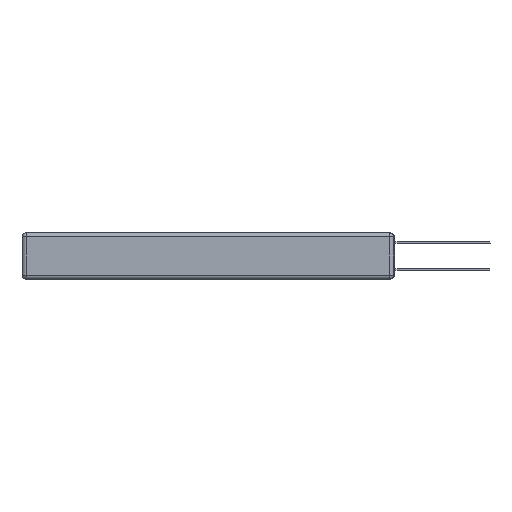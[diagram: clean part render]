
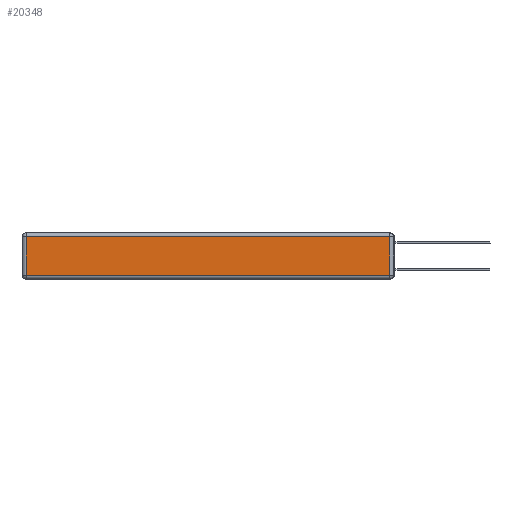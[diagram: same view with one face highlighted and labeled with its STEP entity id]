
A CAD part, left-side view. The second image highlights one B-rep face of the part: STEP entity #20348.
In plain terms, the highlighted planar face has unit normal (-1, 0, 0).
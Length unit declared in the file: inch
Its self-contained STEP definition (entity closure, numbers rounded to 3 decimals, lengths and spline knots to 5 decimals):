
#201 = VERTEX_POINT ( 'NONE', #10310 ) ;
#242 = VECTOR ( 'NONE', #2855, 39.37008 ) ;
#1112 = DIRECTION ( 'NONE',  ( 0., 0., -1. ) ) ;
#1991 = DIRECTION ( 'NONE',  ( 0., -1., 0. ) ) ;
#2254 = DIRECTION ( 'NONE',  ( 0., 0., 1. ) ) ;
#2322 = DIRECTION ( 'NONE',  ( -1., 0., 0. ) ) ;
#2855 = DIRECTION ( 'NONE',  ( 0., 0., 1. ) ) ;
#2873 = CARTESIAN_POINT ( 'NONE',  ( 0., 2.72, -0.343 ) ) ;
#3686 = CARTESIAN_POINT ( 'NONE',  ( 0., 0.03, -0.313 ) ) ;
#3688 = ORIENTED_EDGE ( 'NONE', *, *, #10841, .T. ) ;
#3863 = ORIENTED_EDGE ( 'NONE', *, *, #12484, .T. ) ;
#4446 = EDGE_LOOP ( 'NONE', ( #3863, #12918, #3688, #16856 ) ) ;
#4991 = VECTOR ( 'NONE', #1991, 39.37008 ) ;
#5814 = DIRECTION ( 'NONE',  ( 0., 1., 0. ) ) ;
#9276 = CARTESIAN_POINT ( 'NONE',  ( 0., 2.72, -0.03 ) ) ;
#10310 = CARTESIAN_POINT ( 'NONE',  ( 0., 2.72, -0.313 ) ) ;
#10839 = LINE ( 'NONE', #2873, #19304 ) ;
#10841 = EDGE_CURVE ( 'NONE', #18148, #19157, #12049, .T. ) ;
#12049 = LINE ( 'NONE', #21049, #18689 ) ;
#12332 = PLANE ( 'NONE',  #14252 ) ;
#12484 = EDGE_CURVE ( 'NONE', #201, #20874, #14377, .T. ) ;
#12678 = CARTESIAN_POINT ( 'NONE',  ( 0., 0.03, -0.03 ) ) ;
#12861 = CARTESIAN_POINT ( 'NONE',  ( 0., 0.03, -0.343 ) ) ;
#12918 = ORIENTED_EDGE ( 'NONE', *, *, #17045, .T. ) ;
#14252 = AXIS2_PLACEMENT_3D ( 'NONE', #19153, #2322, #2254 ) ;
#14377 = LINE ( 'NONE', #15380, #4991 ) ;
#15380 = CARTESIAN_POINT ( 'NONE',  ( 0., 0., -0.313 ) ) ;
#16856 = ORIENTED_EDGE ( 'NONE', *, *, #21032, .T. ) ;
#17045 = EDGE_CURVE ( 'NONE', #20874, #18148, #18106, .T. ) ;
#17425 = FACE_OUTER_BOUND ( 'NONE', #4446, .T. ) ;
#18106 = LINE ( 'NONE', #12861, #242 ) ;
#18148 = VERTEX_POINT ( 'NONE', #12678 ) ;
#18689 = VECTOR ( 'NONE', #5814, 39.37008 ) ;
#19153 = CARTESIAN_POINT ( 'NONE',  ( 0., 0., -0.343 ) ) ;
#19157 = VERTEX_POINT ( 'NONE', #9276 ) ;
#19304 = VECTOR ( 'NONE', #1112, 39.37008 ) ;
#20348 = ADVANCED_FACE ( 'NONE', ( #17425 ), #12332, .T. ) ;
#20874 = VERTEX_POINT ( 'NONE', #3686 ) ;
#21032 = EDGE_CURVE ( 'NONE', #19157, #201, #10839, .T. ) ;
#21049 = CARTESIAN_POINT ( 'NONE',  ( 0., 2.75, -0.03 ) ) ;
